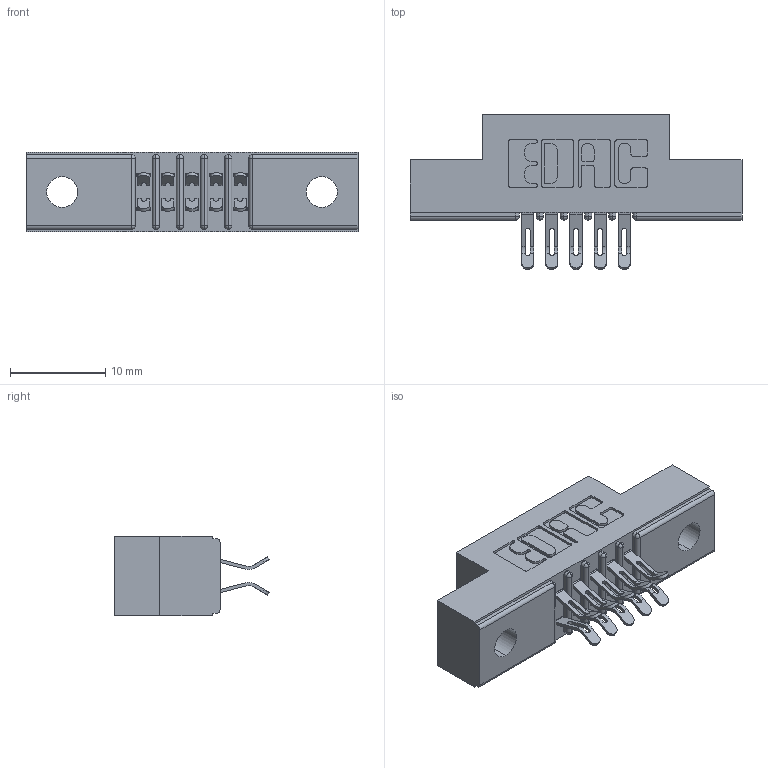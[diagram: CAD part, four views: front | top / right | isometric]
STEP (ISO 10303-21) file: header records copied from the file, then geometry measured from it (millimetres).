
FILE_DESCRIPTION (( 'STEP AP203' ), '1' );
FILE_NAME ('391-010-555-202.STEP', '2018-08-08T16:06:15', ( '' ), ( '' ), 'SwSTEP 2.0', 'SolidWorks 2016', '' );
FILE_SCHEMA (( 'CONFIG_CONTROL_DESIGN' ));
Length unit declared in the file: inch
Products named in the file (3): 341-292-001_341-292-155; 391-010-555-202; 341 Part_.128 (3.25) Dia Mounting Holes
Assembly tree (11 placements, depth 2):
  391-010-555-202
    341 Part_.128 (3.25) Dia Mounting Holes
    341-292-001_341-292-155  x10
Bounding box: 34.92 x 16.31 x 8.38 mm (x, y, z)
Volume: 2007.3 mm3; surface area: 2973.3 mm2
Topology: 11 solids, 11 shells, 896 faces, 2651 edges, 1726 vertices
Faces by surface type: plane 488, cylinder 388, sphere 12, torus 8
Entity records: 11452 total; most frequent: CARTESIAN_POINT 1921, ORIENTED_EDGE 1894, DIRECTION 1881, EDGE_CURVE 947, LINE 709, VECTOR 709, VERTEX_POINT 610, AXIS2_PLACEMENT_3D 586
